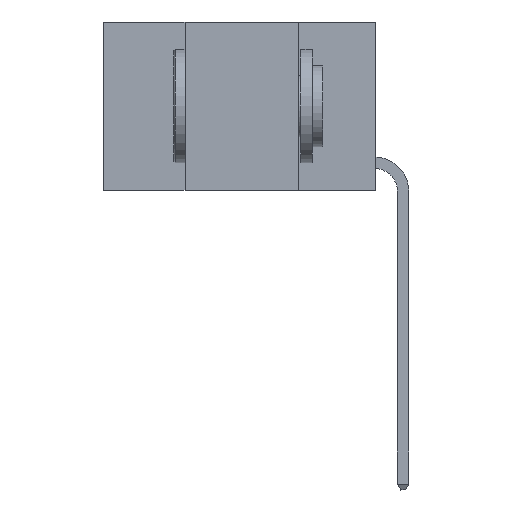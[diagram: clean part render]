
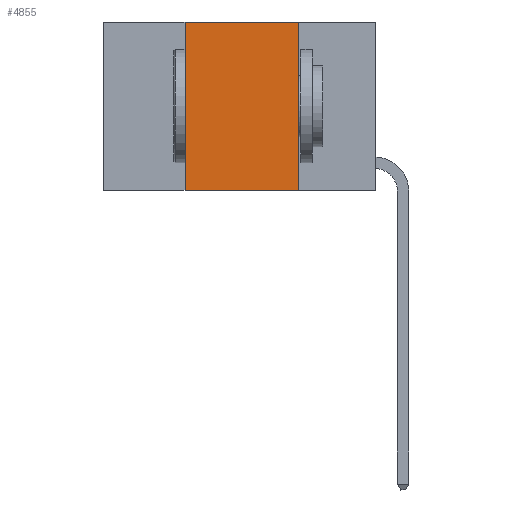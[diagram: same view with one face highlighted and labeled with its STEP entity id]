
A CAD part, left-side view. The second image highlights one B-rep face of the part: STEP entity #4855.
In plain terms, the highlighted planar face has unit normal (-1, 0, 0).
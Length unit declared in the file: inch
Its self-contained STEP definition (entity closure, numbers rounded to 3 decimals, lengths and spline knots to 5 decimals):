
#114 = VERTEX_POINT ( 'NONE', #12283 ) ;
#159 = VECTOR ( 'NONE', #2601, 39.37008 ) ;
#380 = ORIENTED_EDGE ( 'NONE', *, *, #5601, .F. ) ;
#468 = VECTOR ( 'NONE', #5363, 39.37008 ) ;
#819 = CARTESIAN_POINT ( 'NONE',  ( 0., 0.42, -0.37 ) ) ;
#1200 = EDGE_CURVE ( 'NONE', #6797, #10794, #12164, .T. ) ;
#1836 = DIRECTION ( 'NONE',  ( 0., 0., -1. ) ) ;
#1898 = PLANE ( 'NONE',  #12132 ) ;
#2477 = LINE ( 'NONE', #12059, #159 ) ;
#2601 = DIRECTION ( 'NONE',  ( 0., -1., 0. ) ) ;
#3175 = CARTESIAN_POINT ( 'NONE',  ( 0., 0.17, 0. ) ) ;
#3423 = EDGE_CURVE ( 'NONE', #6797, #114, #2477, .T. ) ;
#4090 = VECTOR ( 'NONE', #10306, 39.37008 ) ;
#4190 = ORIENTED_EDGE ( 'NONE', *, *, #11826, .F. ) ;
#4252 = LINE ( 'NONE', #3175, #11370 ) ;
#4662 = CARTESIAN_POINT ( 'NONE',  ( 0., 0.17, 0. ) ) ;
#4816 = DIRECTION ( 'NONE',  ( 1., 0., 0. ) ) ;
#4855 = ADVANCED_FACE ( 'NONE', ( #12241 ), #1898, .F. ) ;
#5363 = DIRECTION ( 'NONE',  ( 0., -1., 0. ) ) ;
#5601 = EDGE_CURVE ( 'NONE', #10794, #12102, #9302, .T. ) ;
#6759 = CARTESIAN_POINT ( 'NONE',  ( 0., 0.42, 0. ) ) ;
#6797 = VERTEX_POINT ( 'NONE', #819 ) ;
#7928 = ORIENTED_EDGE ( 'NONE', *, *, #3423, .T. ) ;
#8919 = DIRECTION ( 'NONE',  ( 0., 0., -1. ) ) ;
#9130 = CARTESIAN_POINT ( 'NONE',  ( 0., 0.42, 0. ) ) ;
#9302 = LINE ( 'NONE', #9999, #468 ) ;
#9445 = CARTESIAN_POINT ( 'NONE',  ( 0., 0.6, 0. ) ) ;
#9999 = CARTESIAN_POINT ( 'NONE',  ( 0., 0.6, 0. ) ) ;
#10306 = DIRECTION ( 'NONE',  ( 0., 0., 1. ) ) ;
#10794 = VERTEX_POINT ( 'NONE', #6759 ) ;
#11221 = EDGE_LOOP ( 'NONE', ( #4190, #380, #11742, #7928 ) ) ;
#11370 = VECTOR ( 'NONE', #8919, 39.37008 ) ;
#11742 = ORIENTED_EDGE ( 'NONE', *, *, #1200, .F. ) ;
#11826 = EDGE_CURVE ( 'NONE', #12102, #114, #4252, .T. ) ;
#12059 = CARTESIAN_POINT ( 'NONE',  ( 0., 0.6, -0.37 ) ) ;
#12102 = VERTEX_POINT ( 'NONE', #4662 ) ;
#12132 = AXIS2_PLACEMENT_3D ( 'NONE', #9445, #4816, #1836 ) ;
#12164 = LINE ( 'NONE', #9130, #4090 ) ;
#12241 = FACE_OUTER_BOUND ( 'NONE', #11221, .T. ) ;
#12283 = CARTESIAN_POINT ( 'NONE',  ( 0., 0.17, -0.37 ) ) ;
